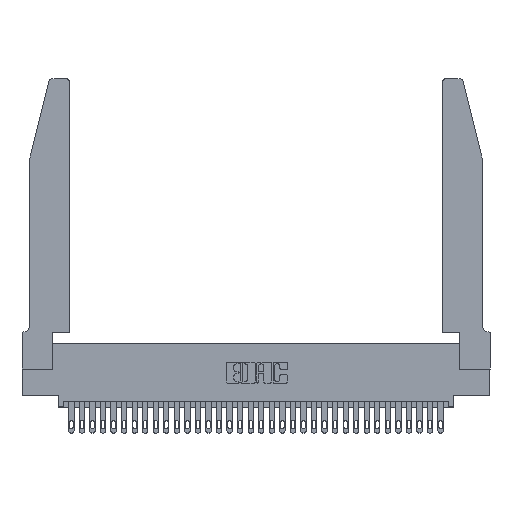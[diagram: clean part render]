
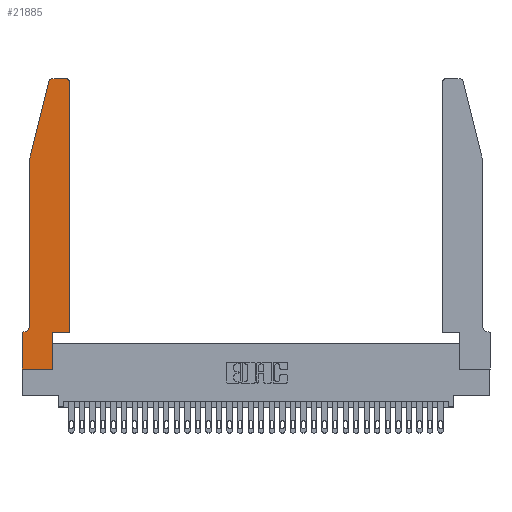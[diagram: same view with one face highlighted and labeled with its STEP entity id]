
A CAD part, top view. The second image highlights one B-rep face of the part: STEP entity #21885.
In plain terms, the highlighted planar face has unit normal (0, 0, 1).
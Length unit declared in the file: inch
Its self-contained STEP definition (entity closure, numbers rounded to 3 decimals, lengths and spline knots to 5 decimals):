
#466 = EDGE_CURVE ( 'NONE', #30654, #14590, #13373, .T. ) ;
#568 = ORIENTED_EDGE ( 'NONE', *, *, #20776, .T. ) ;
#696 = DIRECTION ( 'NONE',  ( 0., -1., 0. ) ) ;
#736 = ORIENTED_EDGE ( 'NONE', *, *, #28522, .T. ) ;
#880 = DIRECTION ( 'NONE',  ( 1., 0., 0. ) ) ;
#904 = VECTOR ( 'NONE', #21057, 39.37008 ) ;
#997 = AXIS2_PLACEMENT_3D ( 'NONE', #21934, #14009, #6097 ) ;
#1001 = LINE ( 'NONE', #8505, #32111 ) ;
#1113 = DIRECTION ( 'NONE',  ( 0., 0., 1. ) ) ;
#1228 = CARTESIAN_POINT ( 'NONE',  ( 0.284, 2.75, 0.37 ) ) ;
#1267 = AXIS2_PLACEMENT_3D ( 'NONE', #20164, #15232, #18089 ) ;
#1825 = DIRECTION ( 'NONE',  ( -1., 0., 0. ) ) ;
#1927 = ORIENTED_EDGE ( 'NONE', *, *, #25716, .T. ) ;
#1981 = CARTESIAN_POINT ( 'NONE',  ( 0.4505, 0.35, 0.37 ) ) ;
#2122 = DIRECTION ( 'NONE',  ( 1., 0., 0. ) ) ;
#2331 = VECTOR ( 'NONE', #1825, 39.37008 ) ;
#2938 = VECTOR ( 'NONE', #2122, 39.37008 ) ;
#3153 = DIRECTION ( 'NONE',  ( 0., 1., 0. ) ) ;
#3231 = AXIS2_PLACEMENT_3D ( 'NONE', #22264, #30150, #14447 ) ;
#3683 = EDGE_CURVE ( 'NONE', #17898, #9168, #14890, .T. ) ;
#4420 = VERTEX_POINT ( 'NONE', #25806 ) ;
#4753 = ORIENTED_EDGE ( 'NONE', *, *, #22360, .T. ) ;
#4779 = CARTESIAN_POINT ( 'NONE',  ( 0., 0.35, 0.37 ) ) ;
#5138 = LINE ( 'NONE', #9923, #2331 ) ;
#5539 = CARTESIAN_POINT ( 'NONE',  ( 0.0755, 2., 0.37 ) ) ;
#5718 = CARTESIAN_POINT ( 'NONE',  ( 0., 0., 0.37 ) ) ;
#5740 = DIRECTION ( 'NONE',  ( 1., 0., 0. ) ) ;
#6097 = DIRECTION ( 'NONE',  ( 1., 0., 0. ) ) ;
#7868 = CARTESIAN_POINT ( 'NONE',  ( 0.0755, 2., 0.37 ) ) ;
#8505 = CARTESIAN_POINT ( 'NONE',  ( 0.4505, 0.35, 0.37 ) ) ;
#8577 = ORIENTED_EDGE ( 'NONE', *, *, #28955, .T. ) ;
#8998 = VECTOR ( 'NONE', #33302, 39.37008 ) ;
#9168 = VERTEX_POINT ( 'NONE', #5539 ) ;
#9437 = EDGE_CURVE ( 'NONE', #25923, #30654, #9924, .T. ) ;
#9816 = CARTESIAN_POINT ( 'NONE',  ( 0.2865, 0.35, 0.37 ) ) ;
#9923 = CARTESIAN_POINT ( 'NONE',  ( 0.0755, 0.35, 0.37 ) ) ;
#9924 = LINE ( 'NONE', #20003, #2938 ) ;
#10174 = ORIENTED_EDGE ( 'NONE', *, *, #28175, .T. ) ;
#10436 = LINE ( 'NONE', #20050, #20323 ) ;
#11193 = ORIENTED_EDGE ( 'NONE', *, *, #31399, .T. ) ;
#12094 = CIRCLE ( 'NONE', #1267, 0.07 ) ;
#13257 = FACE_OUTER_BOUND ( 'NONE', #30590, .T. ) ;
#13323 = CARTESIAN_POINT ( 'NONE',  ( 0., 0., 0.37 ) ) ;
#13373 = LINE ( 'NONE', #17555, #18714 ) ;
#13772 = EDGE_CURVE ( 'NONE', #14709, #28818, #12094, .T. ) ;
#14009 = DIRECTION ( 'NONE',  ( 0., 0., 1. ) ) ;
#14447 = DIRECTION ( 'NONE',  ( 1., 0., 0. ) ) ;
#14590 = VERTEX_POINT ( 'NONE', #9816 ) ;
#14709 = VERTEX_POINT ( 'NONE', #27841 ) ;
#14890 = LINE ( 'NONE', #7868, #904 ) ;
#14943 = VERTEX_POINT ( 'NONE', #1228 ) ;
#15232 = DIRECTION ( 'NONE',  ( 0., 0., -1. ) ) ;
#15422 = VECTOR ( 'NONE', #3153, 39.37008 ) ;
#15592 = AXIS2_PLACEMENT_3D ( 'NONE', #28881, #1113, #880 ) ;
#16720 = CARTESIAN_POINT ( 'NONE',  ( 0.4205, 2.75, 0.37 ) ) ;
#17058 = LINE ( 'NONE', #29305, #15422 ) ;
#17555 = CARTESIAN_POINT ( 'NONE',  ( 0.2865, 0.35, 0.37 ) ) ;
#17898 = VERTEX_POINT ( 'NONE', #32766 ) ;
#18089 = DIRECTION ( 'NONE',  ( -1., 0., 0. ) ) ;
#18714 = VECTOR ( 'NONE', #32885, 39.37008 ) ;
#18812 = ORIENTED_EDGE ( 'NONE', *, *, #21213, .T. ) ;
#19438 = VERTEX_POINT ( 'NONE', #4779 ) ;
#19468 = CIRCLE ( 'NONE', #15592, 0.03 ) ;
#19828 = PLANE ( 'NONE',  #3231 ) ;
#19901 = CARTESIAN_POINT ( 'NONE',  ( 0.0755, 2., 0.37 ) ) ;
#20003 = CARTESIAN_POINT ( 'NONE',  ( 0., 0., 0.37 ) ) ;
#20050 = CARTESIAN_POINT ( 'NONE',  ( 0.2605, 2.75, 0.37 ) ) ;
#20164 = CARTESIAN_POINT ( 'NONE',  ( 0.0055, 0.42, 0.37 ) ) ;
#20285 = VERTEX_POINT ( 'NONE', #16720 ) ;
#20323 = VECTOR ( 'NONE', #30819, 39.37008 ) ;
#20776 = EDGE_CURVE ( 'NONE', #20285, #14943, #10436, .T. ) ;
#20815 = ORIENTED_EDGE ( 'NONE', *, *, #466, .T. ) ;
#21057 = DIRECTION ( 'NONE',  ( -0.239, -0.971, 0. ) ) ;
#21096 = VECTOR ( 'NONE', #696, 39.37008 ) ;
#21213 = EDGE_CURVE ( 'NONE', #14590, #22098, #1001, .T. ) ;
#21885 = ADVANCED_FACE ( 'NONE', ( #13257 ), #19828, .T. ) ;
#21934 = CARTESIAN_POINT ( 'NONE',  ( 0.284, 2.72, 0.37 ) ) ;
#22098 = VERTEX_POINT ( 'NONE', #1981 ) ;
#22264 = CARTESIAN_POINT ( 'NONE',  ( 0., 0.35, 0.37 ) ) ;
#22360 = EDGE_CURVE ( 'NONE', #4420, #20285, #19468, .T. ) ;
#22920 = CARTESIAN_POINT ( 'NONE',  ( 0.2865, 0., 0.37 ) ) ;
#22934 = CIRCLE ( 'NONE', #997, 0.03 ) ;
#24119 = CARTESIAN_POINT ( 'NONE',  ( 0.0055, 0.35, 0.37 ) ) ;
#25716 = EDGE_CURVE ( 'NONE', #9168, #14709, #27479, .T. ) ;
#25806 = CARTESIAN_POINT ( 'NONE',  ( 0.4505, 2.72, 0.37 ) ) ;
#25923 = VERTEX_POINT ( 'NONE', #13323 ) ;
#25985 = ORIENTED_EDGE ( 'NONE', *, *, #3683, .T. ) ;
#27276 = ORIENTED_EDGE ( 'NONE', *, *, #13772, .T. ) ;
#27479 = LINE ( 'NONE', #19901, #8998 ) ;
#27841 = CARTESIAN_POINT ( 'NONE',  ( 0.0755, 0.42, 0.37 ) ) ;
#28175 = EDGE_CURVE ( 'NONE', #22098, #4420, #17058, .T. ) ;
#28522 = EDGE_CURVE ( 'NONE', #28818, #19438, #5138, .T. ) ;
#28818 = VERTEX_POINT ( 'NONE', #24119 ) ;
#28881 = CARTESIAN_POINT ( 'NONE',  ( 0.4205, 2.72, 0.37 ) ) ;
#28955 = EDGE_CURVE ( 'NONE', #14943, #17898, #22934, .T. ) ;
#29305 = CARTESIAN_POINT ( 'NONE',  ( 0.4505, 0.35, 0.37 ) ) ;
#30150 = DIRECTION ( 'NONE',  ( 0., 0., 1. ) ) ;
#30590 = EDGE_LOOP ( 'NONE', ( #568, #8577, #25985, #1927, #27276, #736, #11193, #31570, #20815, #18812, #10174, #4753 ) ) ;
#30654 = VERTEX_POINT ( 'NONE', #22920 ) ;
#30819 = DIRECTION ( 'NONE',  ( -1., 0., 0. ) ) ;
#31355 = LINE ( 'NONE', #5718, #21096 ) ;
#31399 = EDGE_CURVE ( 'NONE', #19438, #25923, #31355, .T. ) ;
#31570 = ORIENTED_EDGE ( 'NONE', *, *, #9437, .T. ) ;
#32111 = VECTOR ( 'NONE', #5740, 39.37008 ) ;
#32766 = CARTESIAN_POINT ( 'NONE',  ( 0.25487, 2.72718, 0.37 ) ) ;
#32885 = DIRECTION ( 'NONE',  ( 0., 1., 0. ) ) ;
#33302 = DIRECTION ( 'NONE',  ( 0., -1., 0. ) ) ;
